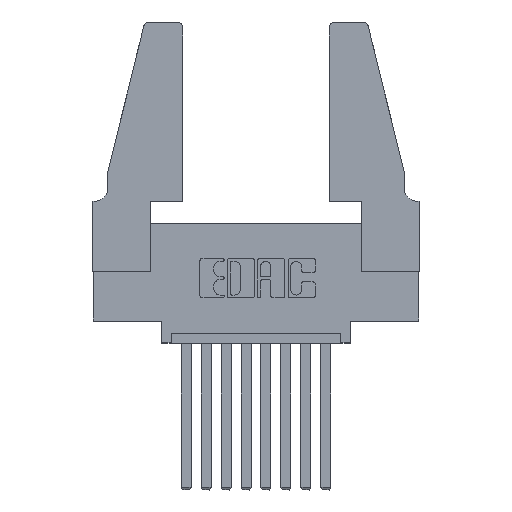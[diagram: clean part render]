
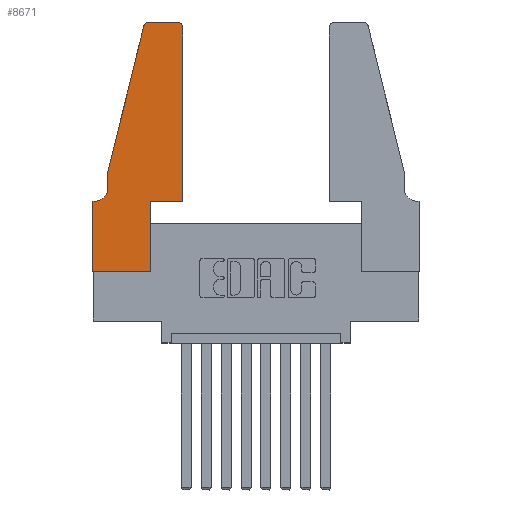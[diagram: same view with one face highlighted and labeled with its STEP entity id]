
A CAD part, top view. The second image highlights one B-rep face of the part: STEP entity #8671.
In plain terms, the highlighted planar face has unit normal (0, 0, 1).
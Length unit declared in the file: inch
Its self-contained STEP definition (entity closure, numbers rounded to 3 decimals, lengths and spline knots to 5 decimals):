
#42 = EDGE_CURVE ( 'NONE', #10567, #9294, #12554, .T. ) ;
#114 = VECTOR ( 'NONE', #2406, 39.37008 ) ;
#167 = AXIS2_PLACEMENT_3D ( 'NONE', #12111, #315, #7154 ) ;
#231 = CARTESIAN_POINT ( 'NONE',  ( 0.4205, 1.22, 0.37 ) ) ;
#268 = DIRECTION ( 'NONE',  ( 1., 0., 0. ) ) ;
#315 = DIRECTION ( 'NONE',  ( 0., 0., 1. ) ) ;
#423 = DIRECTION ( 'NONE',  ( -0.239, -0.971, 0. ) ) ;
#433 = ORIENTED_EDGE ( 'NONE', *, *, #8598, .T. ) ;
#581 = EDGE_CURVE ( 'NONE', #9198, #6662, #6455, .T. ) ;
#608 = CARTESIAN_POINT ( 'NONE',  ( 0.0755, 0.42, 0.37 ) ) ;
#721 = CARTESIAN_POINT ( 'NONE',  ( 0.284, 1.25, 0.37 ) ) ;
#996 = ORIENTED_EDGE ( 'NONE', *, *, #581, .T. ) ;
#1065 = VERTEX_POINT ( 'NONE', #2499 ) ;
#1112 = FACE_OUTER_BOUND ( 'NONE', #3611, .T. ) ;
#1271 = CARTESIAN_POINT ( 'NONE',  ( 0., 0.35, 0.37 ) ) ;
#1298 = VECTOR ( 'NONE', #5282, 39.37008 ) ;
#1332 = CARTESIAN_POINT ( 'NONE',  ( 0.2865, 0.35, 0.37 ) ) ;
#1388 = DIRECTION ( 'NONE',  ( 1., 0., 0. ) ) ;
#1633 = LINE ( 'NONE', #8244, #10541 ) ;
#1669 = AXIS2_PLACEMENT_3D ( 'NONE', #231, #9221, #268 ) ;
#2068 = CARTESIAN_POINT ( 'NONE',  ( 0., 0., 0.37 ) ) ;
#2218 = DIRECTION ( 'NONE',  ( 0., 1., 0. ) ) ;
#2356 = LINE ( 'NONE', #4375, #1298 ) ;
#2406 = DIRECTION ( 'NONE',  ( 0., 1., 0. ) ) ;
#2410 = ORIENTED_EDGE ( 'NONE', *, *, #10471, .T. ) ;
#2478 = ORIENTED_EDGE ( 'NONE', *, *, #2928, .T. ) ;
#2499 = CARTESIAN_POINT ( 'NONE',  ( 0.4205, 1.25, 0.37 ) ) ;
#2593 = ORIENTED_EDGE ( 'NONE', *, *, #8314, .T. ) ;
#2596 = CARTESIAN_POINT ( 'NONE',  ( 0.0055, 0.42, 0.37 ) ) ;
#2782 = CIRCLE ( 'NONE', #8863, 0.07 ) ;
#2928 = EDGE_CURVE ( 'NONE', #8722, #3791, #1633, .T. ) ;
#3029 = VERTEX_POINT ( 'NONE', #721 ) ;
#3414 = CIRCLE ( 'NONE', #1669, 0.03 ) ;
#3483 = VERTEX_POINT ( 'NONE', #5041 ) ;
#3611 = EDGE_LOOP ( 'NONE', ( #2410, #10413, #2478, #433, #12211, #11314, #5431, #996, #5373, #11179, #7270, #2593 ) ) ;
#3763 = LINE ( 'NONE', #9230, #114 ) ;
#3791 = VERTEX_POINT ( 'NONE', #12584 ) ;
#3993 = CARTESIAN_POINT ( 'NONE',  ( 0., 0.35, 0.37 ) ) ;
#4002 = VECTOR ( 'NONE', #11696, 39.37008 ) ;
#4006 = EDGE_CURVE ( 'NONE', #6858, #9090, #2356, .T. ) ;
#4170 = CARTESIAN_POINT ( 'NONE',  ( 0.2605, 1.25, 0.37 ) ) ;
#4375 = CARTESIAN_POINT ( 'NONE',  ( 0.0755, 0.35, 0.37 ) ) ;
#4699 = EDGE_CURVE ( 'NONE', #9090, #9198, #5902, .T. ) ;
#5041 = CARTESIAN_POINT ( 'NONE',  ( 0.4505, 1.22, 0.37 ) ) ;
#5246 = PLANE ( 'NONE',  #9974 ) ;
#5282 = DIRECTION ( 'NONE',  ( -1., 0., 0. ) ) ;
#5373 = ORIENTED_EDGE ( 'NONE', *, *, #7360, .T. ) ;
#5431 = ORIENTED_EDGE ( 'NONE', *, *, #4699, .T. ) ;
#5470 = VECTOR ( 'NONE', #6710, 39.37008 ) ;
#5608 = EDGE_CURVE ( 'NONE', #12570, #6858, #2782, .T. ) ;
#5844 = VECTOR ( 'NONE', #7938, 39.37008 ) ;
#5897 = CARTESIAN_POINT ( 'NONE',  ( 0.2865, 0., 0.37 ) ) ;
#5902 = LINE ( 'NONE', #2068, #11882 ) ;
#6054 = CARTESIAN_POINT ( 'NONE',  ( 0.25487, 1.22718, 0.37 ) ) ;
#6111 = EDGE_CURVE ( 'NONE', #3029, #8722, #7064, .T. ) ;
#6182 = LINE ( 'NONE', #9727, #4002 ) ;
#6204 = CARTESIAN_POINT ( 'NONE',  ( 0.2865, 0.35, 0.37 ) ) ;
#6455 = LINE ( 'NONE', #11556, #9366 ) ;
#6662 = VERTEX_POINT ( 'NONE', #5897 ) ;
#6710 = DIRECTION ( 'NONE',  ( 1., 0., 0. ) ) ;
#6858 = VERTEX_POINT ( 'NONE', #11257 ) ;
#7064 = CIRCLE ( 'NONE', #167, 0.03 ) ;
#7110 = VECTOR ( 'NONE', #2218, 39.37008 ) ;
#7154 = DIRECTION ( 'NONE',  ( 1., 0., 0. ) ) ;
#7256 = DIRECTION ( 'NONE',  ( 0., 0., 1. ) ) ;
#7270 = ORIENTED_EDGE ( 'NONE', *, *, #12406, .T. ) ;
#7360 = EDGE_CURVE ( 'NONE', #6662, #10567, #7730, .T. ) ;
#7730 = LINE ( 'NONE', #1332, #7110 ) ;
#7741 = DIRECTION ( 'NONE',  ( 0., -1., 0. ) ) ;
#7938 = DIRECTION ( 'NONE',  ( -1., 0., 0. ) ) ;
#8244 = CARTESIAN_POINT ( 'NONE',  ( 0.0755, 0.5, 0.37 ) ) ;
#8314 = EDGE_CURVE ( 'NONE', #3483, #1065, #3414, .T. ) ;
#8465 = CARTESIAN_POINT ( 'NONE',  ( 0.4505, 0.35, 0.37 ) ) ;
#8584 = DIRECTION ( 'NONE',  ( 1., 0., 0. ) ) ;
#8598 = EDGE_CURVE ( 'NONE', #3791, #12570, #6182, .T. ) ;
#8671 = ADVANCED_FACE ( 'NONE', ( #1112 ), #5246, .T. ) ;
#8722 = VERTEX_POINT ( 'NONE', #6054 ) ;
#8863 = AXIS2_PLACEMENT_3D ( 'NONE', #2596, #12424, #11312 ) ;
#9090 = VERTEX_POINT ( 'NONE', #3993 ) ;
#9198 = VERTEX_POINT ( 'NONE', #12411 ) ;
#9221 = DIRECTION ( 'NONE',  ( 0., 0., 1. ) ) ;
#9230 = CARTESIAN_POINT ( 'NONE',  ( 0.4505, 0.35, 0.37 ) ) ;
#9294 = VERTEX_POINT ( 'NONE', #8465 ) ;
#9366 = VECTOR ( 'NONE', #8584, 39.37008 ) ;
#9727 = CARTESIAN_POINT ( 'NONE',  ( 0.0755, 0.5, 0.37 ) ) ;
#9974 = AXIS2_PLACEMENT_3D ( 'NONE', #1271, #7256, #1388 ) ;
#10413 = ORIENTED_EDGE ( 'NONE', *, *, #6111, .T. ) ;
#10460 = LINE ( 'NONE', #4170, #5844 ) ;
#10471 = EDGE_CURVE ( 'NONE', #1065, #3029, #10460, .T. ) ;
#10541 = VECTOR ( 'NONE', #423, 39.37008 ) ;
#10567 = VERTEX_POINT ( 'NONE', #6204 ) ;
#11179 = ORIENTED_EDGE ( 'NONE', *, *, #42, .T. ) ;
#11257 = CARTESIAN_POINT ( 'NONE',  ( 0.0055, 0.35, 0.37 ) ) ;
#11312 = DIRECTION ( 'NONE',  ( -1., 0., 0. ) ) ;
#11314 = ORIENTED_EDGE ( 'NONE', *, *, #4006, .T. ) ;
#11556 = CARTESIAN_POINT ( 'NONE',  ( 0., 0., 0.37 ) ) ;
#11696 = DIRECTION ( 'NONE',  ( 0., -1., 0. ) ) ;
#11882 = VECTOR ( 'NONE', #7741, 39.37008 ) ;
#12111 = CARTESIAN_POINT ( 'NONE',  ( 0.284, 1.22, 0.37 ) ) ;
#12211 = ORIENTED_EDGE ( 'NONE', *, *, #5608, .T. ) ;
#12406 = EDGE_CURVE ( 'NONE', #9294, #3483, #3763, .T. ) ;
#12411 = CARTESIAN_POINT ( 'NONE',  ( 0., 0., 0.37 ) ) ;
#12424 = DIRECTION ( 'NONE',  ( 0., 0., -1. ) ) ;
#12554 = LINE ( 'NONE', #12586, #5470 ) ;
#12570 = VERTEX_POINT ( 'NONE', #608 ) ;
#12584 = CARTESIAN_POINT ( 'NONE',  ( 0.0755, 0.5, 0.37 ) ) ;
#12586 = CARTESIAN_POINT ( 'NONE',  ( 0.4505, 0.35, 0.37 ) ) ;
